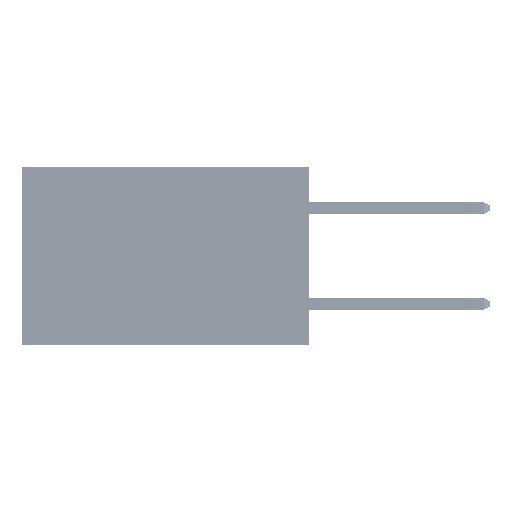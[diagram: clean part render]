
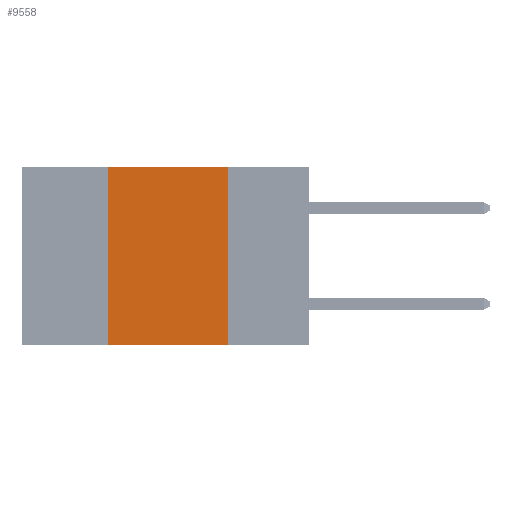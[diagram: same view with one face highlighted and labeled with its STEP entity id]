
A CAD part, left-side view. The second image highlights one B-rep face of the part: STEP entity #9558.
In plain terms, the highlighted planar face has unit normal (-1, 0, 0).
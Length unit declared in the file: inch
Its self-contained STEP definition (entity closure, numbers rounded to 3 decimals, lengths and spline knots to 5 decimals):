
#1017 = LINE ( 'NONE', #8127, #24293 ) ;
#1412 = CARTESIAN_POINT ( 'NONE',  ( 0., 0.6, 0. ) ) ;
#2015 = ORIENTED_EDGE ( 'NONE', *, *, #37173, .F. ) ;
#4193 = CARTESIAN_POINT ( 'NONE',  ( 0., 0.42, 0. ) ) ;
#5032 = PLANE ( 'NONE',  #31232 ) ;
#5043 = VERTEX_POINT ( 'NONE', #24867 ) ;
#6447 = ORIENTED_EDGE ( 'NONE', *, *, #39364, .T. ) ;
#6469 = DIRECTION ( 'NONE',  ( 0., 0., 1. ) ) ;
#7463 = VECTOR ( 'NONE', #6469, 39.37008 ) ;
#8127 = CARTESIAN_POINT ( 'NONE',  ( 0., 0.6, 0. ) ) ;
#9558 = ADVANCED_FACE ( 'NONE', ( #14326 ), #5032, .F. ) ;
#11754 = CARTESIAN_POINT ( 'NONE',  ( 0., 0.6, -0.37 ) ) ;
#13644 = ORIENTED_EDGE ( 'NONE', *, *, #43030, .F. ) ;
#14326 = FACE_OUTER_BOUND ( 'NONE', #46102, .T. ) ;
#15117 = VERTEX_POINT ( 'NONE', #45262 ) ;
#17414 = VERTEX_POINT ( 'NONE', #44017 ) ;
#17453 = EDGE_CURVE ( 'NONE', #31824, #15117, #1017, .T. ) ;
#17695 = CARTESIAN_POINT ( 'NONE',  ( 0., 0.17, 0. ) ) ;
#17726 = CARTESIAN_POINT ( 'NONE',  ( 0., 0.42, 0. ) ) ;
#19087 = DIRECTION ( 'NONE',  ( 0., -1., 0. ) ) ;
#24293 = VECTOR ( 'NONE', #43672, 39.37008 ) ;
#24867 = CARTESIAN_POINT ( 'NONE',  ( 0., 0.42, -0.37 ) ) ;
#31232 = AXIS2_PLACEMENT_3D ( 'NONE', #1412, #40589, #44364 ) ;
#31824 = VERTEX_POINT ( 'NONE', #4193 ) ;
#34390 = LINE ( 'NONE', #17726, #7463 ) ;
#37173 = EDGE_CURVE ( 'NONE', #5043, #31824, #34390, .T. ) ;
#37822 = ORIENTED_EDGE ( 'NONE', *, *, #17453, .F. ) ;
#39118 = LINE ( 'NONE', #17695, #45843 ) ;
#39364 = EDGE_CURVE ( 'NONE', #5043, #17414, #44518, .T. ) ;
#40589 = DIRECTION ( 'NONE',  ( 1., 0., 0. ) ) ;
#43030 = EDGE_CURVE ( 'NONE', #15117, #17414, #39118, .T. ) ;
#43672 = DIRECTION ( 'NONE',  ( 0., -1., 0. ) ) ;
#43923 = VECTOR ( 'NONE', #19087, 39.37008 ) ;
#44017 = CARTESIAN_POINT ( 'NONE',  ( 0., 0.17, -0.37 ) ) ;
#44364 = DIRECTION ( 'NONE',  ( 0., 0., -1. ) ) ;
#44518 = LINE ( 'NONE', #11754, #43923 ) ;
#45262 = CARTESIAN_POINT ( 'NONE',  ( 0., 0.17, 0. ) ) ;
#45843 = VECTOR ( 'NONE', #48507, 39.37008 ) ;
#46102 = EDGE_LOOP ( 'NONE', ( #13644, #37822, #2015, #6447 ) ) ;
#48507 = DIRECTION ( 'NONE',  ( 0., 0., -1. ) ) ;
